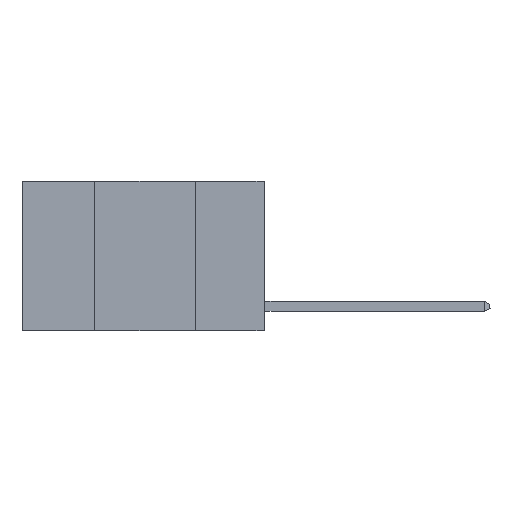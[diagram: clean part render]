
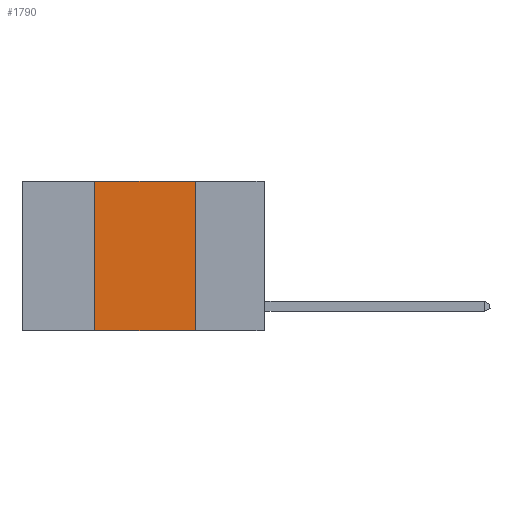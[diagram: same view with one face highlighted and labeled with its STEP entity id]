
A CAD part, left-side view. The second image highlights one B-rep face of the part: STEP entity #1790.
In plain terms, the highlighted planar face has unit normal (-1, 0, 0).
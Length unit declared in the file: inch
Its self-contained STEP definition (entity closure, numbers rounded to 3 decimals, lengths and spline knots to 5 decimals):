
#303 = DIRECTION ( 'NONE',  ( 0., -1., 0. ) ) ;
#571 = ORIENTED_EDGE ( 'NONE', *, *, #17492, .F. ) ;
#761 = CARTESIAN_POINT ( 'NONE',  ( 0., 0.6, -0.37 ) ) ;
#794 = VERTEX_POINT ( 'NONE', #7785 ) ;
#991 = DIRECTION ( 'NONE',  ( 0., -1., 0. ) ) ;
#1790 = ADVANCED_FACE ( 'NONE', ( #12178 ), #22683, .F. ) ;
#1812 = CARTESIAN_POINT ( 'NONE',  ( 0., 0.42, -0.37 ) ) ;
#1841 = VERTEX_POINT ( 'NONE', #1812 ) ;
#2232 = CARTESIAN_POINT ( 'NONE',  ( 0., 0.17, -0.37 ) ) ;
#4135 = DIRECTION ( 'NONE',  ( 0., 0., 1. ) ) ;
#7785 = CARTESIAN_POINT ( 'NONE',  ( 0., 0.42, 0. ) ) ;
#8527 = CARTESIAN_POINT ( 'NONE',  ( 0., 0.17, 0. ) ) ;
#8672 = VECTOR ( 'NONE', #991, 39.37008 ) ;
#8916 = DIRECTION ( 'NONE',  ( 0., 0., -1. ) ) ;
#9014 = LINE ( 'NONE', #20943, #18367 ) ;
#9226 = VERTEX_POINT ( 'NONE', #2232 ) ;
#11745 = ORIENTED_EDGE ( 'NONE', *, *, #15475, .F. ) ;
#12178 = FACE_OUTER_BOUND ( 'NONE', #19899, .T. ) ;
#12969 = CARTESIAN_POINT ( 'NONE',  ( 0., 0.17, 0. ) ) ;
#14031 = DIRECTION ( 'NONE',  ( 1., 0., 0. ) ) ;
#14225 = VECTOR ( 'NONE', #14460, 39.37008 ) ;
#14460 = DIRECTION ( 'NONE',  ( 0., 0., -1. ) ) ;
#15475 = EDGE_CURVE ( 'NONE', #19744, #9226, #21097, .T. ) ;
#15624 = EDGE_CURVE ( 'NONE', #1841, #9226, #16566, .T. ) ;
#16109 = AXIS2_PLACEMENT_3D ( 'NONE', #21406, #14031, #8916 ) ;
#16167 = ORIENTED_EDGE ( 'NONE', *, *, #15624, .T. ) ;
#16566 = LINE ( 'NONE', #761, #8672 ) ;
#16668 = EDGE_CURVE ( 'NONE', #1841, #794, #22023, .T. ) ;
#17492 = EDGE_CURVE ( 'NONE', #794, #19744, #9014, .T. ) ;
#18367 = VECTOR ( 'NONE', #303, 39.37008 ) ;
#19744 = VERTEX_POINT ( 'NONE', #8527 ) ;
#19899 = EDGE_LOOP ( 'NONE', ( #11745, #571, #21979, #16167 ) ) ;
#20886 = VECTOR ( 'NONE', #4135, 39.37008 ) ;
#20943 = CARTESIAN_POINT ( 'NONE',  ( 0., 0.6, 0. ) ) ;
#21097 = LINE ( 'NONE', #12969, #14225 ) ;
#21406 = CARTESIAN_POINT ( 'NONE',  ( 0., 0.6, 0. ) ) ;
#21900 = CARTESIAN_POINT ( 'NONE',  ( 0., 0.42, 0. ) ) ;
#21979 = ORIENTED_EDGE ( 'NONE', *, *, #16668, .F. ) ;
#22023 = LINE ( 'NONE', #21900, #20886 ) ;
#22683 = PLANE ( 'NONE',  #16109 ) ;
